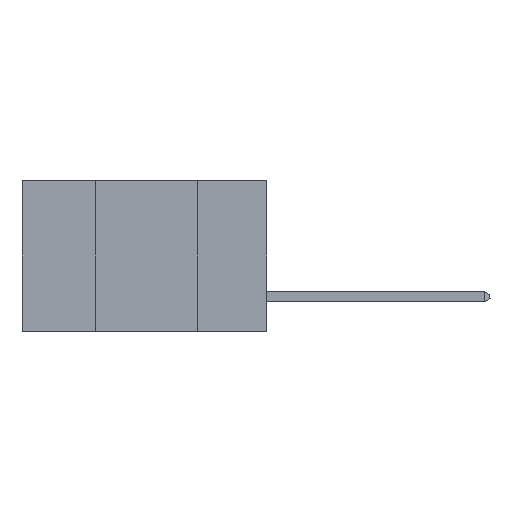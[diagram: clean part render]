
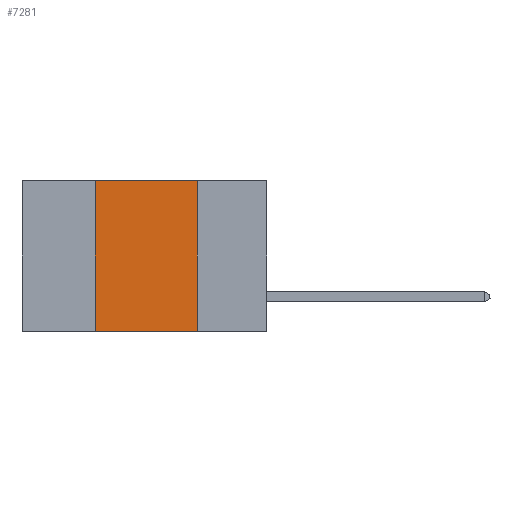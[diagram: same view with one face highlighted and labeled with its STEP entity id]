
A CAD part, left-side view. The second image highlights one B-rep face of the part: STEP entity #7281.
In plain terms, the highlighted planar face has unit normal (-1, 0, 0).
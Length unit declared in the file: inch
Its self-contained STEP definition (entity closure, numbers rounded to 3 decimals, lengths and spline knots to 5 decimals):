
#93 = VERTEX_POINT ( 'NONE', #3118 ) ;
#3015 = PLANE ( 'NONE',  #29799 ) ;
#3118 = CARTESIAN_POINT ( 'NONE',  ( 0., 0.17, -0.37 ) ) ;
#3611 = DIRECTION ( 'NONE',  ( 0., -1., 0. ) ) ;
#5363 = VECTOR ( 'NONE', #19633, 39.37008 ) ;
#7281 = ADVANCED_FACE ( 'NONE', ( #21590 ), #3015, .F. ) ;
#7697 = EDGE_CURVE ( 'NONE', #22528, #93, #12522, .T. ) ;
#8786 = CARTESIAN_POINT ( 'NONE',  ( 0., 0.17, 0. ) ) ;
#10131 = ORIENTED_EDGE ( 'NONE', *, *, #7697, .F. ) ;
#10299 = DIRECTION ( 'NONE',  ( 0., 0., -1. ) ) ;
#11865 = ORIENTED_EDGE ( 'NONE', *, *, #25545, .F. ) ;
#12522 = LINE ( 'NONE', #19430, #5363 ) ;
#12710 = DIRECTION ( 'NONE',  ( 1., 0., 0. ) ) ;
#12793 = LINE ( 'NONE', #27618, #16908 ) ;
#13628 = CARTESIAN_POINT ( 'NONE',  ( 0., 0.42, 0. ) ) ;
#14345 = ORIENTED_EDGE ( 'NONE', *, *, #29552, .F. ) ;
#15861 = VERTEX_POINT ( 'NONE', #26367 ) ;
#16590 = ORIENTED_EDGE ( 'NONE', *, *, #29307, .T. ) ;
#16908 = VECTOR ( 'NONE', #27178, 39.37008 ) ;
#17687 = VECTOR ( 'NONE', #30284, 39.37008 ) ;
#18308 = EDGE_LOOP ( 'NONE', ( #10131, #11865, #14345, #16590 ) ) ;
#19430 = CARTESIAN_POINT ( 'NONE',  ( 0., 0.17, 0. ) ) ;
#19563 = VECTOR ( 'NONE', #3611, 39.37008 ) ;
#19633 = DIRECTION ( 'NONE',  ( 0., 0., -1. ) ) ;
#20335 = LINE ( 'NONE', #13628, #17687 ) ;
#20530 = VERTEX_POINT ( 'NONE', #23333 ) ;
#21590 = FACE_OUTER_BOUND ( 'NONE', #18308, .T. ) ;
#22528 = VERTEX_POINT ( 'NONE', #8786 ) ;
#23333 = CARTESIAN_POINT ( 'NONE',  ( 0., 0.42, -0.37 ) ) ;
#25545 = EDGE_CURVE ( 'NONE', #15861, #22528, #12793, .T. ) ;
#26367 = CARTESIAN_POINT ( 'NONE',  ( 0., 0.42, 0. ) ) ;
#27178 = DIRECTION ( 'NONE',  ( 0., -1., 0. ) ) ;
#27427 = CARTESIAN_POINT ( 'NONE',  ( 0., 0.6, -0.37 ) ) ;
#27618 = CARTESIAN_POINT ( 'NONE',  ( 0., 0.6, 0. ) ) ;
#29307 = EDGE_CURVE ( 'NONE', #20530, #93, #30496, .T. ) ;
#29552 = EDGE_CURVE ( 'NONE', #20530, #15861, #20335, .T. ) ;
#29794 = CARTESIAN_POINT ( 'NONE',  ( 0., 0.6, 0. ) ) ;
#29799 = AXIS2_PLACEMENT_3D ( 'NONE', #29794, #12710, #10299 ) ;
#30284 = DIRECTION ( 'NONE',  ( 0., 0., 1. ) ) ;
#30496 = LINE ( 'NONE', #27427, #19563 ) ;
